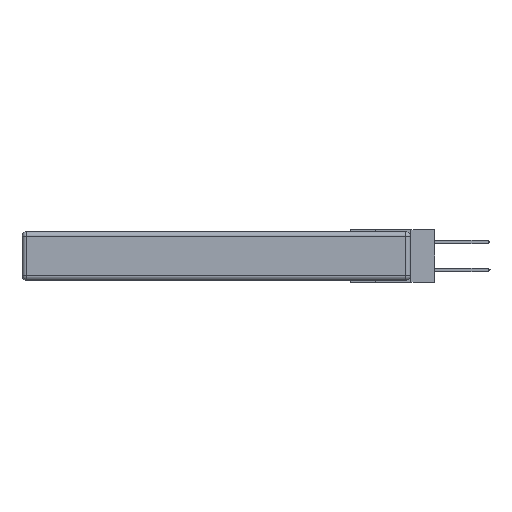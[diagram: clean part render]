
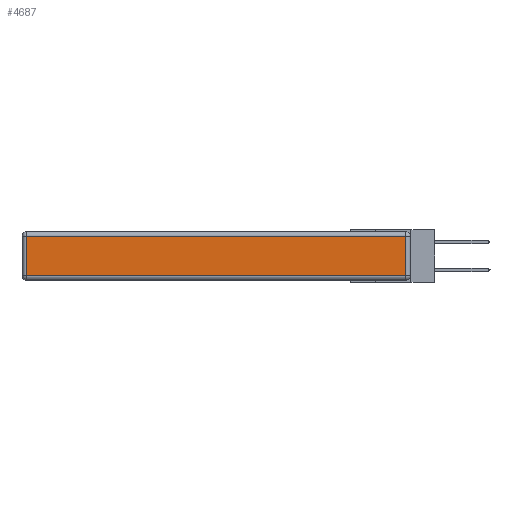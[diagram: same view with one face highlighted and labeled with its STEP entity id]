
A CAD part, left-side view. The second image highlights one B-rep face of the part: STEP entity #4687.
In plain terms, the highlighted planar face has unit normal (-1, 0, 0).
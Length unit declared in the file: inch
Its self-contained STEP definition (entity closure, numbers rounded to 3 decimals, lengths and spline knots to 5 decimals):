
#62 = EDGE_CURVE ( 'NONE', #6399, #8282, #7261, .T. ) ;
#1151 = EDGE_CURVE ( 'NONE', #8282, #4070, #1235, .T. ) ;
#1235 = LINE ( 'NONE', #6538, #1389 ) ;
#1389 = VECTOR ( 'NONE', #2986, 39.37008 ) ;
#2848 = LINE ( 'NONE', #11860, #3564 ) ;
#2986 = DIRECTION ( 'NONE',  ( 0., 0., 1. ) ) ;
#3564 = VECTOR ( 'NONE', #6126, 39.37008 ) ;
#3915 = DIRECTION ( 'NONE',  ( 0., -1., 0. ) ) ;
#3999 = CARTESIAN_POINT ( 'NONE',  ( 0., 0., -0.313 ) ) ;
#4070 = VERTEX_POINT ( 'NONE', #10674 ) ;
#4328 = ORIENTED_EDGE ( 'NONE', *, *, #62, .T. ) ;
#4536 = EDGE_LOOP ( 'NONE', ( #4328, #9737, #5174, #11484 ) ) ;
#4687 = ADVANCED_FACE ( 'NONE', ( #12243 ), #11244, .T. ) ;
#5174 = ORIENTED_EDGE ( 'NONE', *, *, #7219, .T. ) ;
#5283 = LINE ( 'NONE', #6598, #10939 ) ;
#6126 = DIRECTION ( 'NONE',  ( 0., 1., 0. ) ) ;
#6399 = VERTEX_POINT ( 'NONE', #7673 ) ;
#6538 = CARTESIAN_POINT ( 'NONE',  ( 0., 0.03, -0.343 ) ) ;
#6558 = AXIS2_PLACEMENT_3D ( 'NONE', #6863, #7816, #11466 ) ;
#6598 = CARTESIAN_POINT ( 'NONE',  ( 0., 2.72, -0.343 ) ) ;
#6863 = CARTESIAN_POINT ( 'NONE',  ( 0., 0., -0.343 ) ) ;
#6931 = CARTESIAN_POINT ( 'NONE',  ( 0., 2.72, -0.03 ) ) ;
#7219 = EDGE_CURVE ( 'NONE', #4070, #11954, #2848, .T. ) ;
#7261 = LINE ( 'NONE', #3999, #11459 ) ;
#7594 = DIRECTION ( 'NONE',  ( 0., 0., -1. ) ) ;
#7673 = CARTESIAN_POINT ( 'NONE',  ( 0., 2.72, -0.313 ) ) ;
#7816 = DIRECTION ( 'NONE',  ( -1., 0., 0. ) ) ;
#8282 = VERTEX_POINT ( 'NONE', #9104 ) ;
#8638 = EDGE_CURVE ( 'NONE', #11954, #6399, #5283, .T. ) ;
#9104 = CARTESIAN_POINT ( 'NONE',  ( 0., 0.03, -0.313 ) ) ;
#9737 = ORIENTED_EDGE ( 'NONE', *, *, #1151, .T. ) ;
#10674 = CARTESIAN_POINT ( 'NONE',  ( 0., 0.03, -0.03 ) ) ;
#10939 = VECTOR ( 'NONE', #7594, 39.37008 ) ;
#11244 = PLANE ( 'NONE',  #6558 ) ;
#11459 = VECTOR ( 'NONE', #3915, 39.37008 ) ;
#11466 = DIRECTION ( 'NONE',  ( 0., 0., 1. ) ) ;
#11484 = ORIENTED_EDGE ( 'NONE', *, *, #8638, .T. ) ;
#11860 = CARTESIAN_POINT ( 'NONE',  ( 0., 2.75, -0.03 ) ) ;
#11954 = VERTEX_POINT ( 'NONE', #6931 ) ;
#12243 = FACE_OUTER_BOUND ( 'NONE', #4536, .T. ) ;
